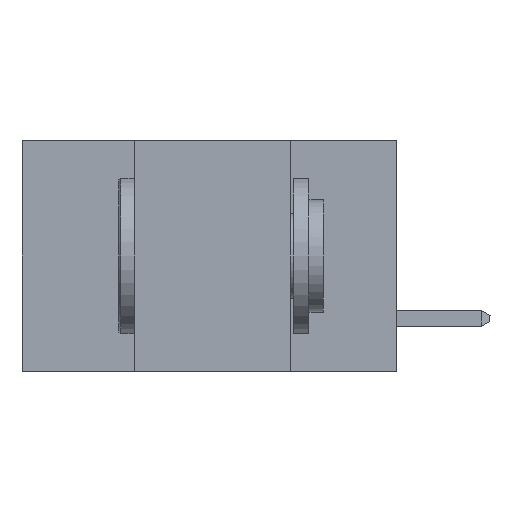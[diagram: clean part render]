
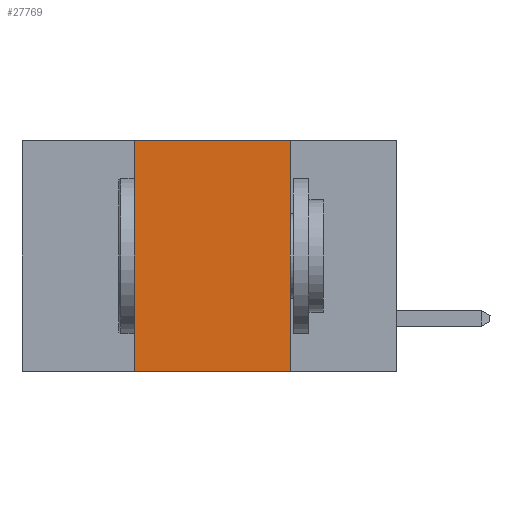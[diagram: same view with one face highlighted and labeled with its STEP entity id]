
A CAD part, left-side view. The second image highlights one B-rep face of the part: STEP entity #27769.
In plain terms, the highlighted planar face has unit normal (-1, 0, 0).
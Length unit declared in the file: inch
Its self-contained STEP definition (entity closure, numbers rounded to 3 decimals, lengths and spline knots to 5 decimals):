
#211 = LINE ( 'NONE', #19311, #15451 ) ;
#1238 = AXIS2_PLACEMENT_3D ( 'NONE', #23589, #1859, #23490 ) ;
#1436 = ORIENTED_EDGE ( 'NONE', *, *, #4115, .F. ) ;
#1859 = DIRECTION ( 'NONE',  ( 1., 0., 0. ) ) ;
#2151 = LINE ( 'NONE', #17229, #22583 ) ;
#2553 = EDGE_CURVE ( 'NONE', #6928, #21726, #21332, .T. ) ;
#3555 = FACE_OUTER_BOUND ( 'NONE', #29356, .T. ) ;
#3677 = CARTESIAN_POINT ( 'NONE',  ( 0., 0.42, 0. ) ) ;
#4115 = EDGE_CURVE ( 'NONE', #16441, #6928, #29379, .T. ) ;
#4781 = ORIENTED_EDGE ( 'NONE', *, *, #2553, .F. ) ;
#6871 = PLANE ( 'NONE',  #1238 ) ;
#6928 = VERTEX_POINT ( 'NONE', #3677 ) ;
#7428 = ORIENTED_EDGE ( 'NONE', *, *, #20056, .F. ) ;
#12094 = DIRECTION ( 'NONE',  ( 0., 0., -1. ) ) ;
#13584 = CARTESIAN_POINT ( 'NONE',  ( 0., 0.17, -0.37 ) ) ;
#13902 = EDGE_CURVE ( 'NONE', #16441, #30141, #2151, .T. ) ;
#15211 = DIRECTION ( 'NONE',  ( 0., 0., 1. ) ) ;
#15451 = VECTOR ( 'NONE', #12094, 39.37008 ) ;
#15505 = CARTESIAN_POINT ( 'NONE',  ( 0., 0.42, -0.37 ) ) ;
#16031 = ORIENTED_EDGE ( 'NONE', *, *, #13902, .T. ) ;
#16441 = VERTEX_POINT ( 'NONE', #15505 ) ;
#17229 = CARTESIAN_POINT ( 'NONE',  ( 0., 0.6, -0.37 ) ) ;
#19311 = CARTESIAN_POINT ( 'NONE',  ( 0., 0.17, 0. ) ) ;
#20056 = EDGE_CURVE ( 'NONE', #21726, #30141, #211, .T. ) ;
#21332 = LINE ( 'NONE', #28430, #22090 ) ;
#21726 = VERTEX_POINT ( 'NONE', #23991 ) ;
#22090 = VECTOR ( 'NONE', #30806, 39.37008 ) ;
#22248 = CARTESIAN_POINT ( 'NONE',  ( 0., 0.42, 0. ) ) ;
#22583 = VECTOR ( 'NONE', #24012, 39.37008 ) ;
#23081 = VECTOR ( 'NONE', #15211, 39.37008 ) ;
#23490 = DIRECTION ( 'NONE',  ( 0., 0., -1. ) ) ;
#23589 = CARTESIAN_POINT ( 'NONE',  ( 0., 0.6, 0. ) ) ;
#23991 = CARTESIAN_POINT ( 'NONE',  ( 0., 0.17, 0. ) ) ;
#24012 = DIRECTION ( 'NONE',  ( 0., -1., 0. ) ) ;
#27769 = ADVANCED_FACE ( 'NONE', ( #3555 ), #6871, .F. ) ;
#28430 = CARTESIAN_POINT ( 'NONE',  ( 0., 0.6, 0. ) ) ;
#29356 = EDGE_LOOP ( 'NONE', ( #7428, #4781, #1436, #16031 ) ) ;
#29379 = LINE ( 'NONE', #22248, #23081 ) ;
#30141 = VERTEX_POINT ( 'NONE', #13584 ) ;
#30806 = DIRECTION ( 'NONE',  ( 0., -1., 0. ) ) ;
